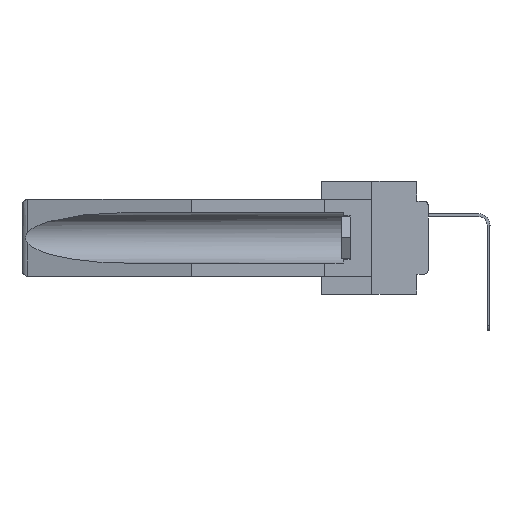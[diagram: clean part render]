
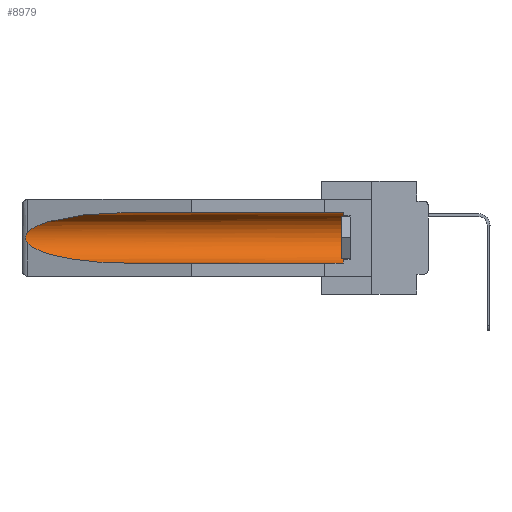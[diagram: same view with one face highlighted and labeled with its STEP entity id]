
A CAD part, left-side view. The second image highlights one B-rep face of the part: STEP entity #8979.
In plain terms, the highlighted cylindrical face has radius 2.857 mm (diameter 5.715 mm), a partial arc.
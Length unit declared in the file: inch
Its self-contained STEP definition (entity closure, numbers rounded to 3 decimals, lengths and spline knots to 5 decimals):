
#86 = CARTESIAN_POINT ( 'NONE',  ( 0.2673, 1.5327, -0.16383 ) ) ;
#208 = AXIS2_PLACEMENT_3D ( 'NONE', #9238, #24236, #31950 ) ;
#238 = CARTESIAN_POINT ( 'NONE',  ( 0.155, 1.07973, -0.284 ) ) ;
#537 = ORIENTED_EDGE ( 'NONE', *, *, #27307, .T. ) ;
#1324 = EDGE_CURVE ( 'NONE', #13293, #21544, #4095, .T. ) ;
#2708 = CARTESIAN_POINT ( 'NONE',  ( 0.26537, 1.52718, -0.14972 ) ) ;
#3267 = ORIENTED_EDGE ( 'NONE', *, *, #1324, .T. ) ;
#4095 = LINE ( 'NONE', #13915, #5694 ) ;
#5694 = VECTOR ( 'NONE', #26602, 39.37008 ) ;
#6163 = VERTEX_POINT ( 'NONE', #24891 ) ;
#6583 = AXIS2_PLACEMENT_3D ( 'NONE', #28294, #30535, #12756 ) ;
#7379 = VERTEX_POINT ( 'NONE', #24601 ) ;
#7629 =( BOUNDED_CURVE ( )  B_SPLINE_CURVE ( 3, ( #11648, #9104, #31835, #16699 ),
 .UNSPECIFIED., .F., .F. ) 
 B_SPLINE_CURVE_WITH_KNOTS ( ( 4, 4 ),
 ( 4.71239, 6.08839 ),
 .UNSPECIFIED. ) 
 CURVE ( )  GEOMETRIC_REPRESENTATION_ITEM ( )  RATIONAL_B_SPLINE_CURVE ( ( 1., 0.848, 0.848, 1. ) ) 
 REPRESENTATION_ITEM ( '' )  );
#8216 = B_SPLINE_CURVE_WITH_KNOTS ( 'NONE', 3,
 ( #2708, #20390, #17723, #86, #10128, #25128, #10456, #25562, #15178, #20277 ),
 .UNSPECIFIED., .F., .F.,
 ( 4, 2, 2, 2, 4 ),
 ( 0., 0.00029, 0.00058, 0.00087, 0.00117 ),
 .UNSPECIFIED. ) ;
#8454 = FACE_OUTER_BOUND ( 'NONE', #14656, .T. ) ;
#8979 = ADVANCED_FACE ( 'NONE', ( #8454 ), #25425, .F. ) ;
#9104 = CARTESIAN_POINT ( 'NONE',  ( 0.21114, 1.30732, -0.059 ) ) ;
#9238 = CARTESIAN_POINT ( 'NONE',  ( 0.155, -0.30754, -0.1715 ) ) ;
#10128 = CARTESIAN_POINT ( 'NONE',  ( 0.2675, 1.53308, -0.16763 ) ) ;
#10456 = CARTESIAN_POINT ( 'NONE',  ( 0.2673, 1.53269, -0.17917 ) ) ;
#10485 = DIRECTION ( 'NONE',  ( 0., 1., 0. ) ) ;
#10692 = EDGE_CURVE ( 'NONE', #6163, #13293, #29590, .T. ) ;
#11216 = CARTESIAN_POINT ( 'NONE',  ( 0.21114, 1.30732, -0.284 ) ) ;
#11648 = CARTESIAN_POINT ( 'NONE',  ( 0.155, 1.07973, -0.059 ) ) ;
#12756 = DIRECTION ( 'NONE',  ( 0., 0., 1. ) ) ;
#12964 = VERTEX_POINT ( 'NONE', #238 ) ;
#13293 = VERTEX_POINT ( 'NONE', #28492 ) ;
#13465 =( BOUNDED_CURVE ( )  B_SPLINE_CURVE ( 3, ( #31836, #19262, #11216, #26651 ),
 .UNSPECIFIED., .F., .F. ) 
 B_SPLINE_CURVE_WITH_KNOTS ( ( 4, 4 ),
 ( 0.1948, 1.5708 ),
 .UNSPECIFIED. ) 
 CURVE ( )  GEOMETRIC_REPRESENTATION_ITEM ( )  RATIONAL_B_SPLINE_CURVE ( ( 1., 0.848, 0.848, 1. ) ) 
 REPRESENTATION_ITEM ( '' )  );
#13915 = CARTESIAN_POINT ( 'NONE',  ( 0.155, -0.30754, -0.059 ) ) ;
#14656 = EDGE_LOOP ( 'NONE', ( #537, #22134, #25435, #23151, #14698, #3267 ) ) ;
#14698 = ORIENTED_EDGE ( 'NONE', *, *, #10692, .T. ) ;
#15178 = CARTESIAN_POINT ( 'NONE',  ( 0.26597, 1.5296, -0.19026 ) ) ;
#16699 = CARTESIAN_POINT ( 'NONE',  ( 0.26537, 1.52718, -0.14972 ) ) ;
#17389 = EDGE_CURVE ( 'NONE', #19542, #7379, #8216, .T. ) ;
#17576 = CARTESIAN_POINT ( 'NONE',  ( 0.26537, 1.52718, -0.14972 ) ) ;
#17723 = CARTESIAN_POINT ( 'NONE',  ( 0.26654, 1.53092, -0.15636 ) ) ;
#18458 = CARTESIAN_POINT ( 'NONE',  ( 0.155, 1.07973, -0.059 ) ) ;
#18761 = EDGE_CURVE ( 'NONE', #6163, #12964, #22221, .T. ) ;
#19262 = CARTESIAN_POINT ( 'NONE',  ( 0.25451, 1.48313, -0.24835 ) ) ;
#19542 = VERTEX_POINT ( 'NONE', #17576 ) ;
#20277 = CARTESIAN_POINT ( 'NONE',  ( 0.26537, 1.52718, -0.19328 ) ) ;
#20390 = CARTESIAN_POINT ( 'NONE',  ( 0.26597, 1.52961, -0.15275 ) ) ;
#21025 = EDGE_CURVE ( 'NONE', #7379, #12964, #13465, .T. ) ;
#21544 = VERTEX_POINT ( 'NONE', #18458 ) ;
#22134 = ORIENTED_EDGE ( 'NONE', *, *, #17389, .T. ) ;
#22221 = LINE ( 'NONE', #22835, #23778 ) ;
#22835 = CARTESIAN_POINT ( 'NONE',  ( 0.155, -0.30754, -0.284 ) ) ;
#23151 = ORIENTED_EDGE ( 'NONE', *, *, #18761, .F. ) ;
#23778 = VECTOR ( 'NONE', #10485, 39.37008 ) ;
#24236 = DIRECTION ( 'NONE',  ( 0., 1., 0. ) ) ;
#24601 = CARTESIAN_POINT ( 'NONE',  ( 0.26537, 1.52718, -0.19328 ) ) ;
#24891 = CARTESIAN_POINT ( 'NONE',  ( 0.155, 0.126, -0.284 ) ) ;
#25128 = CARTESIAN_POINT ( 'NONE',  ( 0.2675, 1.53308, -0.17534 ) ) ;
#25425 = CYLINDRICAL_SURFACE ( 'NONE', #208, 0.1125 ) ;
#25435 = ORIENTED_EDGE ( 'NONE', *, *, #21025, .T. ) ;
#25562 = CARTESIAN_POINT ( 'NONE',  ( 0.26655, 1.53094, -0.18657 ) ) ;
#26602 = DIRECTION ( 'NONE',  ( 0., 1., 0. ) ) ;
#26651 = CARTESIAN_POINT ( 'NONE',  ( 0.155, 1.07973, -0.284 ) ) ;
#27307 = EDGE_CURVE ( 'NONE', #21544, #19542, #7629, .T. ) ;
#28294 = CARTESIAN_POINT ( 'NONE',  ( 0.155, 0.126, -0.1715 ) ) ;
#28492 = CARTESIAN_POINT ( 'NONE',  ( 0.155, 0.126, -0.059 ) ) ;
#29590 = CIRCLE ( 'NONE', #6583, 0.1125 ) ;
#30535 = DIRECTION ( 'NONE',  ( 0., -1., 0. ) ) ;
#31836 = CARTESIAN_POINT ( 'NONE',  ( 0.26537, 1.52718, -0.19328 ) ) ;
#31835 = CARTESIAN_POINT ( 'NONE',  ( 0.25451, 1.48313, -0.09465 ) ) ;
#31950 = DIRECTION ( 'NONE',  ( 0., 0., 1. ) ) ;
